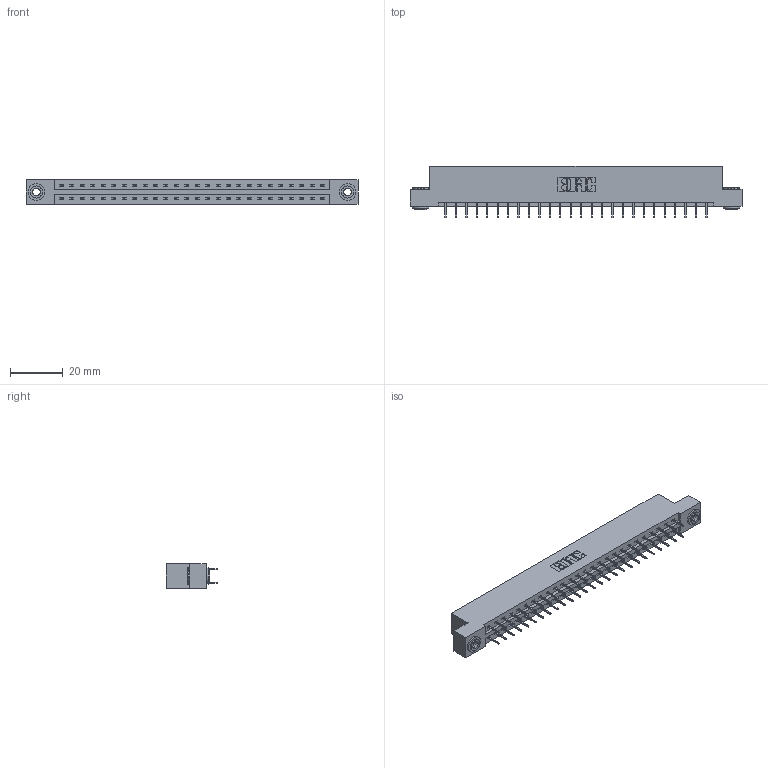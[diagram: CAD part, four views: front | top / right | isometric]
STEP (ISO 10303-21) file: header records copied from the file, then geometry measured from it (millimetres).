
FILE_DESCRIPTION (( 'STEP AP203' ), '1' );
FILE_NAME ('387-052-524-203.STEP', '2018-09-20T10:10:49', ( '' ), ( '' ), 'SwSTEP 2.0', 'SolidWorks 2016', '' );
FILE_SCHEMA (( 'CONFIG_CONTROL_DESIGN' ));
Length unit declared in the file: inch
Products named in the file (4): 337 Part_Flush Mounting Lugs - 0.156 Dia-TH; 345-292-001_345-293-124; 345-250-002_345-250-002-102; 387-052-524-203
Assembly tree (55 placements, depth 2):
  387-052-524-203
    337 Part_Flush Mounting Lugs - 0.156 Dia-TH
    345-292-001_345-293-124  x52
    345-250-002_345-250-002-102  x2
Bounding box: 126.03 x 19.69 x 9.4 mm (x, y, z)
Volume: 13010.3 mm3; surface area: 14533.4 mm2
Topology: 55 solids, 55 shells, 3168 faces, 8967 edges, 5766 vertices
Faces by surface type: plane 2368, cylinder 792, cone 8
Entity records: 22952 total; most frequent: CARTESIAN_POINT 3853, ORIENTED_EDGE 3782, DIRECTION 3341, EDGE_CURVE 1891, LINE 1743, VECTOR 1743, VERTEX_POINT 1254, AXIS2_PLACEMENT_3D 799
